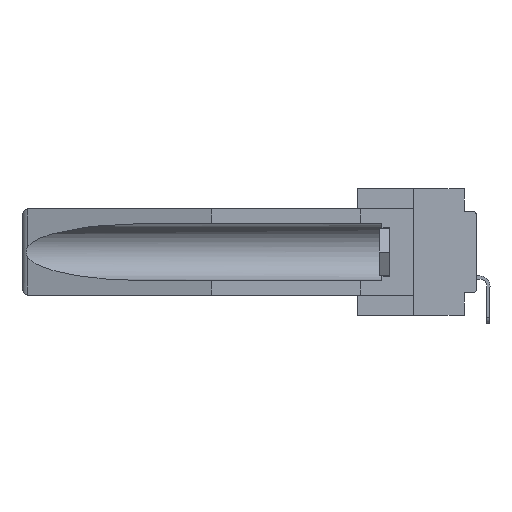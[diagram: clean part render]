
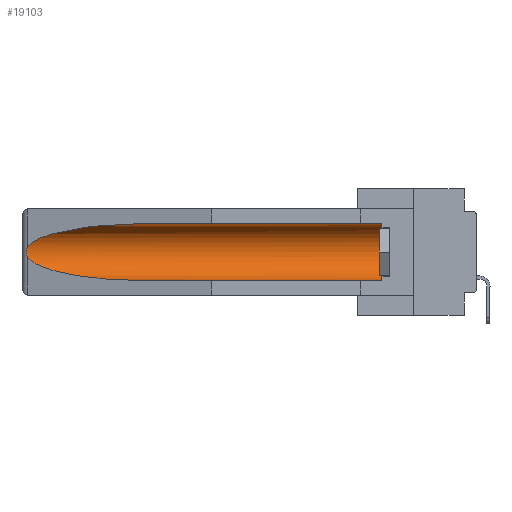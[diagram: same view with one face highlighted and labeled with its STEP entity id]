
A CAD part, left-side view. The second image highlights one B-rep face of the part: STEP entity #19103.
In plain terms, the highlighted cylindrical face has radius 2.857 mm (diameter 5.715 mm), a partial arc.
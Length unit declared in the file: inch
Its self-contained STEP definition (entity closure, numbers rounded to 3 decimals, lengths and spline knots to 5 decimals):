
#284 = VERTEX_POINT ( 'NONE', #22386 ) ;
#632 = CARTESIAN_POINT ( 'NONE',  ( 0.2673, 1.5327, -0.16383 ) ) ;
#675 = DIRECTION ( 'NONE',  ( 0., 1., 0. ) ) ;
#2593 = CARTESIAN_POINT ( 'NONE',  ( 0.2673, 1.53269, -0.17917 ) ) ;
#2785 = CARTESIAN_POINT ( 'NONE',  ( 0.155, 1.07973, -0.284 ) ) ;
#3324 = VERTEX_POINT ( 'NONE', #17401 ) ;
#3349 = VERTEX_POINT ( 'NONE', #15260 ) ;
#4428 = DIRECTION ( 'NONE',  ( 0., 1., 0. ) ) ;
#6435 = ORIENTED_EDGE ( 'NONE', *, *, #27024, .F. ) ;
#6638 =( BOUNDED_CURVE ( )  B_SPLINE_CURVE ( 3, ( #22901, #16238, #25155, #16917 ),
 .UNSPECIFIED., .F., .F. ) 
 B_SPLINE_CURVE_WITH_KNOTS ( ( 4, 4 ),
 ( 0.1948, 1.5708 ),
 .UNSPECIFIED. ) 
 CURVE ( )  GEOMETRIC_REPRESENTATION_ITEM ( )  RATIONAL_B_SPLINE_CURVE ( ( 1., 0.848, 0.848, 1. ) ) 
 REPRESENTATION_ITEM ( '' )  );
#6846 = CARTESIAN_POINT ( 'NONE',  ( 0.26537, 1.52718, -0.14972 ) ) ;
#7103 = ORIENTED_EDGE ( 'NONE', *, *, #28210, .T. ) ;
#7293 = AXIS2_PLACEMENT_3D ( 'NONE', #19989, #26954, #15882 ) ;
#9211 = CARTESIAN_POINT ( 'NONE',  ( 0.155, 0.126, -0.059 ) ) ;
#9391 = CARTESIAN_POINT ( 'NONE',  ( 0.26537, 1.52718, -0.19328 ) ) ;
#10489 = ORIENTED_EDGE ( 'NONE', *, *, #25791, .T. ) ;
#13745 = CARTESIAN_POINT ( 'NONE',  ( 0.2675, 1.53308, -0.16763 ) ) ;
#13925 = CARTESIAN_POINT ( 'NONE',  ( 0.155, 1.07973, -0.059 ) ) ;
#13938 = EDGE_CURVE ( 'NONE', #3349, #20395, #6638, .T. ) ;
#14442 = EDGE_CURVE ( 'NONE', #17971, #3324, #27302, .T. ) ;
#14797 = CARTESIAN_POINT ( 'NONE',  ( 0.155, 0.126, -0.284 ) ) ;
#15211 = B_SPLINE_CURVE_WITH_KNOTS ( 'NONE', 3,
 ( #6846, #22660, #27144, #632, #13745, #15896, #2593, #22546, #22744, #9391 ),
 .UNSPECIFIED., .F., .F.,
 ( 4, 2, 2, 2, 4 ),
 ( 0., 0.00029, 0.00058, 0.00087, 0.00117 ),
 .UNSPECIFIED. ) ;
#15260 = CARTESIAN_POINT ( 'NONE',  ( 0.26537, 1.52718, -0.19328 ) ) ;
#15416 = CYLINDRICAL_SURFACE ( 'NONE', #26876, 0.1125 ) ;
#15882 = DIRECTION ( 'NONE',  ( 0., 0., 1. ) ) ;
#15896 = CARTESIAN_POINT ( 'NONE',  ( 0.2675, 1.53308, -0.17534 ) ) ;
#16238 = CARTESIAN_POINT ( 'NONE',  ( 0.25451, 1.48313, -0.24835 ) ) ;
#16917 = CARTESIAN_POINT ( 'NONE',  ( 0.155, 1.07973, -0.284 ) ) ;
#17401 = CARTESIAN_POINT ( 'NONE',  ( 0.155, 1.07973, -0.059 ) ) ;
#17604 = CARTESIAN_POINT ( 'NONE',  ( 0.155, -0.30754, -0.284 ) ) ;
#17738 = ORIENTED_EDGE ( 'NONE', *, *, #14442, .T. ) ;
#17804 = VECTOR ( 'NONE', #26922, 39.37008 ) ;
#17971 = VERTEX_POINT ( 'NONE', #9211 ) ;
#18219 = CARTESIAN_POINT ( 'NONE',  ( 0.25451, 1.48313, -0.09465 ) ) ;
#19103 = ADVANCED_FACE ( 'NONE', ( #23139 ), #15416, .F. ) ;
#19989 = CARTESIAN_POINT ( 'NONE',  ( 0.155, 0.126, -0.1715 ) ) ;
#20043 = DIRECTION ( 'NONE',  ( 0., 0., 1. ) ) ;
#20330 = CARTESIAN_POINT ( 'NONE',  ( 0.155, -0.30754, -0.1715 ) ) ;
#20395 = VERTEX_POINT ( 'NONE', #2785 ) ;
#20462 = CARTESIAN_POINT ( 'NONE',  ( 0.21114, 1.30732, -0.059 ) ) ;
#20857 = CARTESIAN_POINT ( 'NONE',  ( 0.26537, 1.52718, -0.14972 ) ) ;
#20890 = CIRCLE ( 'NONE', #7293, 0.1125 ) ;
#21514 = EDGE_LOOP ( 'NONE', ( #27824, #10489, #27023, #6435, #7103, #17738 ) ) ;
#21549 = EDGE_CURVE ( 'NONE', #3324, #284, #25240, .T. ) ;
#22386 = CARTESIAN_POINT ( 'NONE',  ( 0.26537, 1.52718, -0.14972 ) ) ;
#22546 = CARTESIAN_POINT ( 'NONE',  ( 0.26655, 1.53094, -0.18657 ) ) ;
#22660 = CARTESIAN_POINT ( 'NONE',  ( 0.26597, 1.52961, -0.15275 ) ) ;
#22744 = CARTESIAN_POINT ( 'NONE',  ( 0.26597, 1.5296, -0.19026 ) ) ;
#22901 = CARTESIAN_POINT ( 'NONE',  ( 0.26537, 1.52718, -0.19328 ) ) ;
#23139 = FACE_OUTER_BOUND ( 'NONE', #21514, .T. ) ;
#23791 = LINE ( 'NONE', #17604, #17804 ) ;
#24914 = VERTEX_POINT ( 'NONE', #14797 ) ;
#25155 = CARTESIAN_POINT ( 'NONE',  ( 0.21114, 1.30732, -0.284 ) ) ;
#25240 =( BOUNDED_CURVE ( )  B_SPLINE_CURVE ( 3, ( #13925, #20462, #18219, #20857 ),
 .UNSPECIFIED., .F., .F. ) 
 B_SPLINE_CURVE_WITH_KNOTS ( ( 4, 4 ),
 ( 4.71239, 6.08839 ),
 .UNSPECIFIED. ) 
 CURVE ( )  GEOMETRIC_REPRESENTATION_ITEM ( )  RATIONAL_B_SPLINE_CURVE ( ( 1., 0.848, 0.848, 1. ) ) 
 REPRESENTATION_ITEM ( '' )  );
#25570 = VECTOR ( 'NONE', #675, 39.37008 ) ;
#25791 = EDGE_CURVE ( 'NONE', #284, #3349, #15211, .T. ) ;
#26876 = AXIS2_PLACEMENT_3D ( 'NONE', #20330, #4428, #20043 ) ;
#26922 = DIRECTION ( 'NONE',  ( 0., 1., 0. ) ) ;
#26954 = DIRECTION ( 'NONE',  ( 0., -1., 0. ) ) ;
#27023 = ORIENTED_EDGE ( 'NONE', *, *, #13938, .T. ) ;
#27024 = EDGE_CURVE ( 'NONE', #24914, #20395, #23791, .T. ) ;
#27144 = CARTESIAN_POINT ( 'NONE',  ( 0.26654, 1.53092, -0.15636 ) ) ;
#27302 = LINE ( 'NONE', #27891, #25570 ) ;
#27824 = ORIENTED_EDGE ( 'NONE', *, *, #21549, .T. ) ;
#27891 = CARTESIAN_POINT ( 'NONE',  ( 0.155, -0.30754, -0.059 ) ) ;
#28210 = EDGE_CURVE ( 'NONE', #24914, #17971, #20890, .T. ) ;
